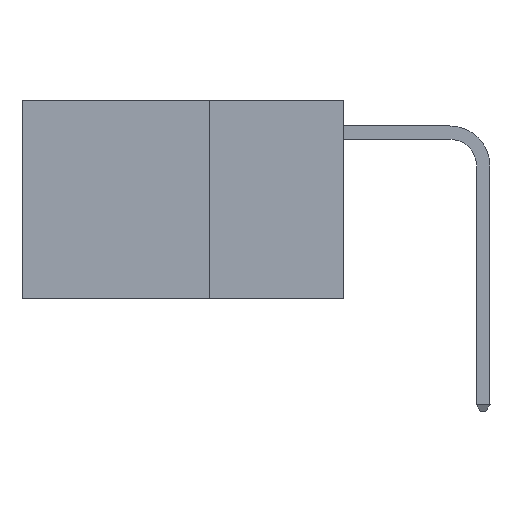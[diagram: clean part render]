
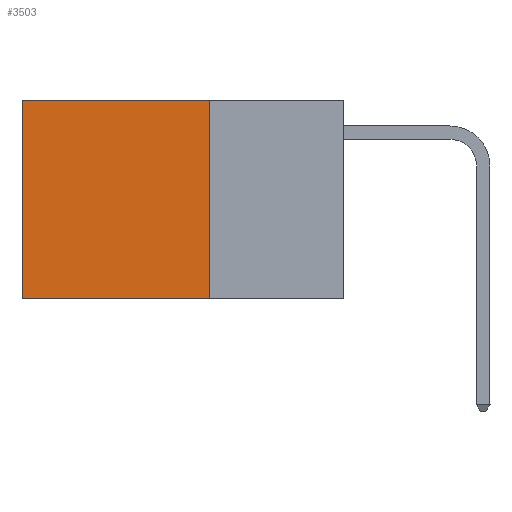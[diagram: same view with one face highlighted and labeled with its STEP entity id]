
A CAD part, left-side view. The second image highlights one B-rep face of the part: STEP entity #3503.
In plain terms, the highlighted planar face has unit normal (-1, 0, 0).
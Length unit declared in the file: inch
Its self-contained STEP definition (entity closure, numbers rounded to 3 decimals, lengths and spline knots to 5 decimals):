
#52 = VECTOR ( 'NONE', #13920, 39.37008 ) ;
#600 = CARTESIAN_POINT ( 'NONE',  ( 0.2625, 0.25, 0. ) ) ;
#1933 = EDGE_LOOP ( 'NONE', ( #9417, #5400, #6633, #21897 ) ) ;
#2127 = FACE_OUTER_BOUND ( 'NONE', #1933, .T. ) ;
#3503 = ADVANCED_FACE ( 'NONE', ( #2127 ), #8487, .F. ) ;
#5394 = DIRECTION ( 'NONE',  ( 0., 1., 0. ) ) ;
#5400 = ORIENTED_EDGE ( 'NONE', *, *, #23881, .F. ) ;
#6633 = ORIENTED_EDGE ( 'NONE', *, *, #14640, .F. ) ;
#6981 = DIRECTION ( 'NONE',  ( 0., 0., -1. ) ) ;
#7529 = VERTEX_POINT ( 'NONE', #20235 ) ;
#8229 = VECTOR ( 'NONE', #6981, 39.37008 ) ;
#8487 = PLANE ( 'NONE',  #20771 ) ;
#8834 = DIRECTION ( 'NONE',  ( 0., 0., -1. ) ) ;
#9417 = ORIENTED_EDGE ( 'NONE', *, *, #21804, .T. ) ;
#9585 = CARTESIAN_POINT ( 'NONE',  ( 0.2625, 0.25, 0. ) ) ;
#10691 = LINE ( 'NONE', #22026, #52 ) ;
#11096 = CARTESIAN_POINT ( 'NONE',  ( 0.2625, 0.6, 0. ) ) ;
#13586 = EDGE_CURVE ( 'NONE', #20124, #18919, #19416, .T. ) ;
#13858 = DIRECTION ( 'NONE',  ( 0., 0., -1. ) ) ;
#13920 = DIRECTION ( 'NONE',  ( 0., 1., 0. ) ) ;
#14640 = EDGE_CURVE ( 'NONE', #20124, #7529, #20951, .T. ) ;
#14653 = DIRECTION ( 'NONE',  ( 1., 0., 0. ) ) ;
#14708 = CARTESIAN_POINT ( 'NONE',  ( 0.2625, 0.25, 0. ) ) ;
#14899 = VECTOR ( 'NONE', #8834, 39.37008 ) ;
#18919 = VERTEX_POINT ( 'NONE', #25504 ) ;
#18944 = LINE ( 'NONE', #11096, #8229 ) ;
#19157 = VERTEX_POINT ( 'NONE', #20237 ) ;
#19416 = LINE ( 'NONE', #9585, #24840 ) ;
#20124 = VERTEX_POINT ( 'NONE', #600 ) ;
#20235 = CARTESIAN_POINT ( 'NONE',  ( 0.2625, 0.25, -0.37 ) ) ;
#20237 = CARTESIAN_POINT ( 'NONE',  ( 0.2625, 0.6, -0.37 ) ) ;
#20771 = AXIS2_PLACEMENT_3D ( 'NONE', #14708, #14653, #13858 ) ;
#20951 = LINE ( 'NONE', #22989, #14899 ) ;
#21804 = EDGE_CURVE ( 'NONE', #18919, #19157, #18944, .T. ) ;
#21897 = ORIENTED_EDGE ( 'NONE', *, *, #13586, .T. ) ;
#22026 = CARTESIAN_POINT ( 'NONE',  ( 0.2625, 0.25, -0.37 ) ) ;
#22989 = CARTESIAN_POINT ( 'NONE',  ( 0.2625, 0.25, 0. ) ) ;
#23881 = EDGE_CURVE ( 'NONE', #7529, #19157, #10691, .T. ) ;
#24840 = VECTOR ( 'NONE', #5394, 39.37008 ) ;
#25504 = CARTESIAN_POINT ( 'NONE',  ( 0.2625, 0.6, 0. ) ) ;
